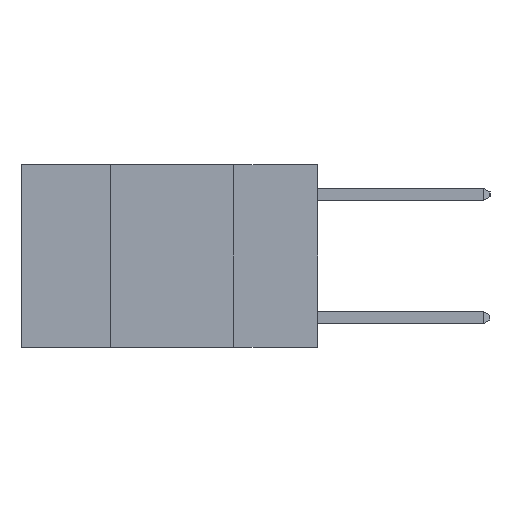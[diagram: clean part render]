
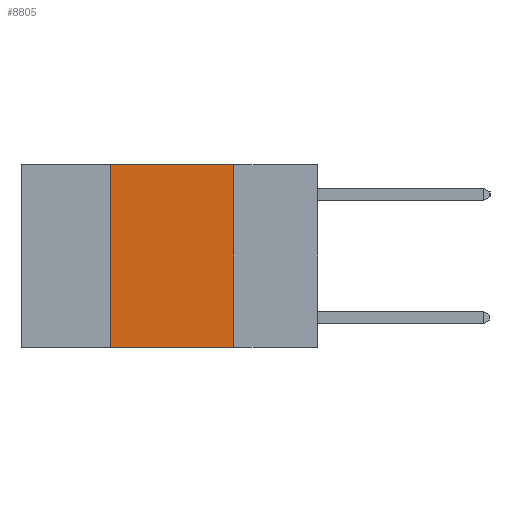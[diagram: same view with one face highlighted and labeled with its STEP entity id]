
A CAD part, left-side view. The second image highlights one B-rep face of the part: STEP entity #8805.
In plain terms, the highlighted planar face has unit normal (-1, 0, 0).
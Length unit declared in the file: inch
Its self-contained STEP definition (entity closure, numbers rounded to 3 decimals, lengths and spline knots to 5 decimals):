
#583 = EDGE_LOOP ( 'NONE', ( #7395, #5593, #922, #3558 ) ) ;
#825 = CARTESIAN_POINT ( 'NONE',  ( 0., 0.42, 0. ) ) ;
#864 = DIRECTION ( 'NONE',  ( 0., -1., 0. ) ) ;
#922 = ORIENTED_EDGE ( 'NONE', *, *, #4368, .F. ) ;
#1290 = LINE ( 'NONE', #5681, #10313 ) ;
#1823 = VERTEX_POINT ( 'NONE', #9688 ) ;
#2094 = DIRECTION ( 'NONE',  ( 0., 0., -1. ) ) ;
#2188 = DIRECTION ( 'NONE',  ( 0., -1., 0. ) ) ;
#2492 = VECTOR ( 'NONE', #5956, 39.37008 ) ;
#3202 = EDGE_CURVE ( 'NONE', #5725, #1823, #1290, .T. ) ;
#3558 = ORIENTED_EDGE ( 'NONE', *, *, #7423, .T. ) ;
#4150 = VERTEX_POINT ( 'NONE', #8221 ) ;
#4245 = FACE_OUTER_BOUND ( 'NONE', #583, .T. ) ;
#4368 = EDGE_CURVE ( 'NONE', #4150, #5725, #7192, .T. ) ;
#4381 = EDGE_CURVE ( 'NONE', #1823, #4504, #4859, .T. ) ;
#4504 = VERTEX_POINT ( 'NONE', #8890 ) ;
#4756 = CARTESIAN_POINT ( 'NONE',  ( 0., 0.6, 0. ) ) ;
#4859 = LINE ( 'NONE', #8617, #9224 ) ;
#5563 = PLANE ( 'NONE',  #8876 ) ;
#5593 = ORIENTED_EDGE ( 'NONE', *, *, #3202, .F. ) ;
#5681 = CARTESIAN_POINT ( 'NONE',  ( 0., 0.6, 0. ) ) ;
#5725 = VERTEX_POINT ( 'NONE', #825 ) ;
#5956 = DIRECTION ( 'NONE',  ( 0., 0., 1. ) ) ;
#7192 = LINE ( 'NONE', #11093, #2492 ) ;
#7385 = DIRECTION ( 'NONE',  ( 1., 0., 0. ) ) ;
#7395 = ORIENTED_EDGE ( 'NONE', *, *, #4381, .F. ) ;
#7423 = EDGE_CURVE ( 'NONE', #4150, #4504, #10613, .T. ) ;
#7750 = DIRECTION ( 'NONE',  ( 0., 0., -1. ) ) ;
#8092 = VECTOR ( 'NONE', #864, 39.37008 ) ;
#8221 = CARTESIAN_POINT ( 'NONE',  ( 0., 0.42, -0.37 ) ) ;
#8617 = CARTESIAN_POINT ( 'NONE',  ( 0., 0.17, 0. ) ) ;
#8805 = ADVANCED_FACE ( 'NONE', ( #4245 ), #5563, .F. ) ;
#8876 = AXIS2_PLACEMENT_3D ( 'NONE', #4756, #7385, #2094 ) ;
#8890 = CARTESIAN_POINT ( 'NONE',  ( 0., 0.17, -0.37 ) ) ;
#9224 = VECTOR ( 'NONE', #7750, 39.37008 ) ;
#9688 = CARTESIAN_POINT ( 'NONE',  ( 0., 0.17, 0. ) ) ;
#10313 = VECTOR ( 'NONE', #2188, 39.37008 ) ;
#10613 = LINE ( 'NONE', #11235, #8092 ) ;
#11093 = CARTESIAN_POINT ( 'NONE',  ( 0., 0.42, 0. ) ) ;
#11235 = CARTESIAN_POINT ( 'NONE',  ( 0., 0.6, -0.37 ) ) ;
